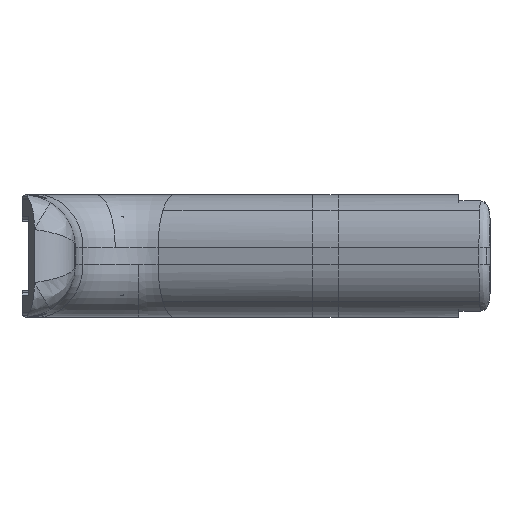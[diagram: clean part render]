
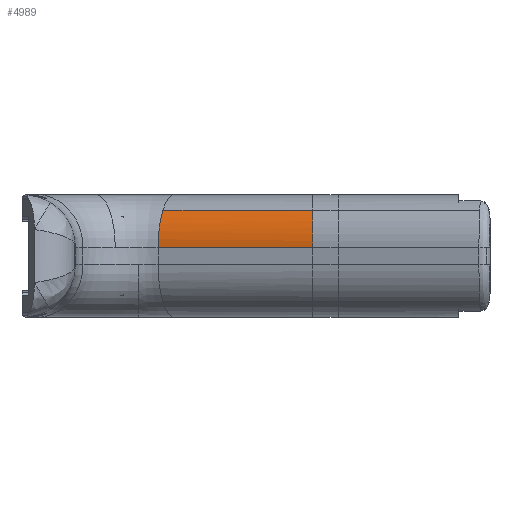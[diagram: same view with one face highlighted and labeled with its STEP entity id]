
A CAD part, left-side view. The second image highlights one B-rep face of the part: STEP entity #4989.
In plain terms, the highlighted cylindrical face has radius 12.5 mm (diameter 25 mm), a partial arc.
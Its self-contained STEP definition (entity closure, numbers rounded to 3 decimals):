
#76 = ORIENTED_EDGE ( 'NONE', *, *, #20253, .T. ) ;
#292 = VERTEX_POINT ( 'NONE', #15858 ) ;
#1926 = AXIS2_PLACEMENT_3D ( 'NONE', #13755, #18365, #20005 ) ;
#2022 = AXIS2_PLACEMENT_3D ( 'NONE', #2870, #6047, #10572 ) ;
#2662 = CYLINDRICAL_SURFACE ( 'NONE', #2022, 12.5 ) ;
#2870 = CARTESIAN_POINT ( 'NONE',  ( -62.55, -12.565, -17.5 ) ) ;
#3815 = VERTEX_POINT ( 'NONE', #9300 ) ;
#4111 = FACE_OUTER_BOUND ( 'NONE', #6741, .T. ) ;
#4989 = ADVANCED_FACE ( 'NONE', ( #4111 ), #2662, .T. ) ;
#5152 = CARTESIAN_POINT ( 'NONE',  ( -77.94, -19.479, -17.5 ) ) ;
#5566 = CARTESIAN_POINT ( 'NONE',  ( -77.94, -19.479, -14.14 ) ) ;
#6047 = DIRECTION ( 'NONE',  ( 0.309, 0.951, 0. ) ) ;
#6077 = CARTESIAN_POINT ( 'NONE',  ( -70.957, -9.834, -8.661 ) ) ;
#6691 = CARTESIAN_POINT ( 'NONE',  ( -74.439, -8.703, -17.5 ) ) ;
#6741 = EDGE_LOOP ( 'NONE', ( #19824, #10444, #76, #16422 ) ) ;
#7715 = DIRECTION ( 'NONE',  ( 0.309, 0.951, 0. ) ) ;
#8635 = CARTESIAN_POINT ( 'NONE',  ( -76.588, -19.479, -11.037 ) ) ;
#8877 = CARTESIAN_POINT ( 'NONE',  ( -77.94, -19.479, -17.5 ) ) ;
#9300 = CARTESIAN_POINT ( 'NONE',  ( -74.091, -19.479, -8.661 ) ) ;
#10444 = ORIENTED_EDGE ( 'NONE', *, *, #10606, .T. ) ;
#10467 = VECTOR ( 'NONE', #16335, 1000. ) ;
#10572 = DIRECTION ( 'NONE',  ( -0.672, 0.219, 0.707 ) ) ;
#10606 = EDGE_CURVE ( 'NONE', #3815, #14853, #20134, .T. ) ;
#11615 = EDGE_CURVE ( 'NONE', #292, #19359, #12464, .T. ) ;
#11732 = VECTOR ( 'NONE', #7715, 1000. ) ;
#12464 = LINE ( 'NONE', #6691, #10467 ) ;
#12789 = EDGE_CURVE ( 'NONE', #3815, #19359, #16407, .T. ) ;
#12954 = CARTESIAN_POINT ( 'NONE',  ( -74.091, -19.479, -8.661 ) ) ;
#13755 = CARTESIAN_POINT ( 'NONE',  ( -54.134, 13.337, -17.5 ) ) ;
#14853 = VERTEX_POINT ( 'NONE', #16201 ) ;
#15858 = CARTESIAN_POINT ( 'NONE',  ( -66.022, 17.2, -17.5 ) ) ;
#16201 = CARTESIAN_POINT ( 'NONE',  ( -62.54, 16.069, -8.661 ) ) ;
#16335 = DIRECTION ( 'NONE',  ( -0.309, -0.951, 0. ) ) ;
#16407 =( BOUNDED_CURVE ( )  B_SPLINE_CURVE ( 3, ( #12954, #8635, #5566, #5152 ),
 .UNSPECIFIED., .F., .F. ) 
 B_SPLINE_CURVE_WITH_KNOTS ( ( 4, 4 ),
 ( 5.498, 6.283 ),
 .UNSPECIFIED. ) 
 CURVE ( )  GEOMETRIC_REPRESENTATION_ITEM ( )  RATIONAL_B_SPLINE_CURVE ( ( 1., 0.949, 0.949, 1. ) ) 
 REPRESENTATION_ITEM ( '' )  );
#16422 = ORIENTED_EDGE ( 'NONE', *, *, #11615, .T. ) ;
#17986 = CIRCLE ( 'NONE', #1926, 12.5 ) ;
#18365 = DIRECTION ( 'NONE',  ( -0.309, -0.951, 0. ) ) ;
#19359 = VERTEX_POINT ( 'NONE', #8877 ) ;
#19824 = ORIENTED_EDGE ( 'NONE', *, *, #12789, .F. ) ;
#20005 = DIRECTION ( 'NONE',  ( 0., 0., 1. ) ) ;
#20134 = LINE ( 'NONE', #6077, #11732 ) ;
#20253 = EDGE_CURVE ( 'NONE', #14853, #292, #17986, .T. ) ;
